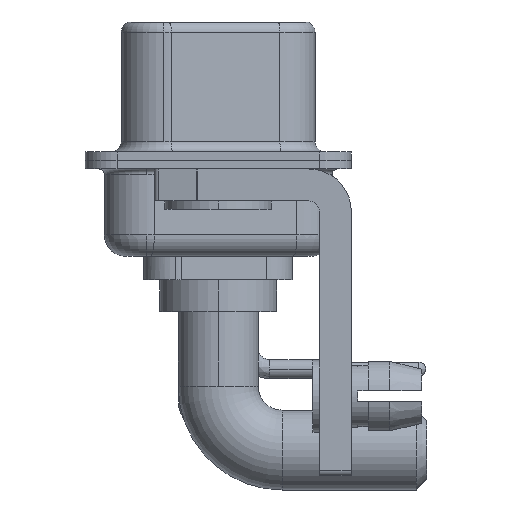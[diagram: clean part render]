
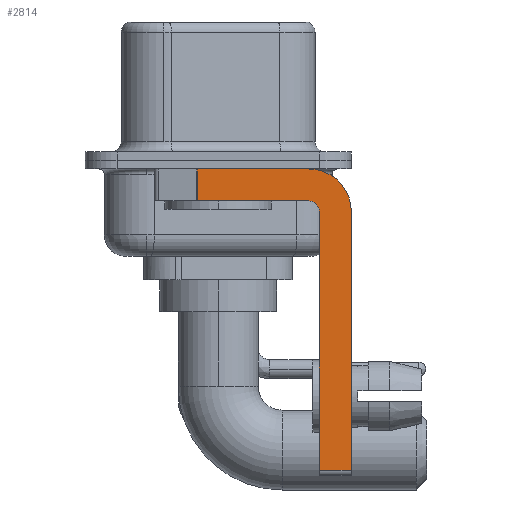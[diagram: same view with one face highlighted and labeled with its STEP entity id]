
A CAD part, left-side view. The second image highlights one B-rep face of the part: STEP entity #2814.
In plain terms, the highlighted planar face has unit normal (-1, 0, 0).
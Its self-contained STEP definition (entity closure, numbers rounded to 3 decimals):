
#138 = CARTESIAN_POINT ( 'NONE',  ( -2.9, -4.25, -1.9 ) ) ;
#366 = VERTEX_POINT ( 'NONE', #13145 ) ;
#1314 = EDGE_CURVE ( 'NONE', #11396, #16834, #12410, .T. ) ;
#1599 = VECTOR ( 'NONE', #16602, 1000. ) ;
#1922 = ORIENTED_EDGE ( 'NONE', *, *, #1314, .F. ) ;
#2042 = DIRECTION ( 'NONE',  ( -1., 0., 0. ) ) ;
#2145 = ORIENTED_EDGE ( 'NONE', *, *, #15794, .T. ) ;
#2553 = DIRECTION ( 'NONE',  ( 0., 0., -1. ) ) ;
#2814 = ADVANCED_FACE ( 'NONE', ( #3043 ), #17117, .F. ) ;
#2923 = CARTESIAN_POINT ( 'NONE',  ( -2.9, -4.75, -2.4 ) ) ;
#3043 = FACE_OUTER_BOUND ( 'NONE', #11314, .T. ) ;
#3869 = DIRECTION ( 'NONE',  ( 0., 0., 1. ) ) ;
#4342 = EDGE_CURVE ( 'NONE', #366, #18215, #15462, .T. ) ;
#4359 = LINE ( 'NONE', #24455, #23652 ) ;
#4376 = ORIENTED_EDGE ( 'NONE', *, *, #16772, .T. ) ;
#4397 = CARTESIAN_POINT ( 'NONE',  ( -2.9, -6.25, -2.4 ) ) ;
#5272 = CARTESIAN_POINT ( 'NONE',  ( -2.9, -4.25, -2.4 ) ) ;
#6816 = CIRCLE ( 'NONE', #10605, 0.5 ) ;
#7728 = EDGE_CURVE ( 'NONE', #23266, #24314, #14425, .T. ) ;
#7977 = DIRECTION ( 'NONE',  ( 0., 0., -1. ) ) ;
#9319 = VECTOR ( 'NONE', #7977, 1000. ) ;
#9496 = VECTOR ( 'NONE', #2553, 1000. ) ;
#9555 = CARTESIAN_POINT ( 'NONE',  ( -2.9, 0.978, -1.9 ) ) ;
#9765 = CARTESIAN_POINT ( 'NONE',  ( -2.9, -6.25, -14.55 ) ) ;
#10085 = DIRECTION ( 'NONE',  ( 0., 0., 1. ) ) ;
#10206 = ORIENTED_EDGE ( 'NONE', *, *, #22269, .F. ) ;
#10605 = AXIS2_PLACEMENT_3D ( 'NONE', #22157, #2042, #10085 ) ;
#11314 = EDGE_LOOP ( 'NONE', ( #15581, #4376, #1922, #10206, #14686, #2145, #24865, #20052 ) ) ;
#11396 = VERTEX_POINT ( 'NONE', #138 ) ;
#11513 = CARTESIAN_POINT ( 'NONE',  ( -2.9, -4.75, -14.8 ) ) ;
#11521 = CARTESIAN_POINT ( 'NONE',  ( -2.9, 0.978, -1.9 ) ) ;
#11612 = DIRECTION ( 'NONE',  ( 1., 0., 0. ) ) ;
#11923 = CARTESIAN_POINT ( 'NONE',  ( -2.9, -4.25, -14.55 ) ) ;
#12410 = LINE ( 'NONE', #14649, #1599 ) ;
#13058 = DIRECTION ( 'NONE',  ( 0., 0., -1. ) ) ;
#13145 = CARTESIAN_POINT ( 'NONE',  ( -2.9, -4.75, -14.55 ) ) ;
#13555 = AXIS2_PLACEMENT_3D ( 'NONE', #15718, #21760, #23703 ) ;
#14024 = LINE ( 'NONE', #9555, #9319 ) ;
#14383 = CARTESIAN_POINT ( 'NONE',  ( -2.9, -6.25, -2.4 ) ) ;
#14425 = LINE ( 'NONE', #4397, #9496 ) ;
#14466 = VECTOR ( 'NONE', #3869, 1000. ) ;
#14649 = CARTESIAN_POINT ( 'NONE',  ( -2.9, -4.25, -1.9 ) ) ;
#14686 = ORIENTED_EDGE ( 'NONE', *, *, #4342, .F. ) ;
#15462 = LINE ( 'NONE', #11513, #14466 ) ;
#15581 = ORIENTED_EDGE ( 'NONE', *, *, #18548, .F. ) ;
#15718 = CARTESIAN_POINT ( 'NONE',  ( -2.9, -4.25, -2.4 ) ) ;
#15794 = EDGE_CURVE ( 'NONE', #366, #24314, #17681, .T. ) ;
#16602 = DIRECTION ( 'NONE',  ( 0., 1., 0. ) ) ;
#16772 = EDGE_CURVE ( 'NONE', #24052, #16834, #14024, .T. ) ;
#16834 = VERTEX_POINT ( 'NONE', #11521 ) ;
#17117 = PLANE ( 'NONE',  #19473 ) ;
#17681 = LINE ( 'NONE', #11923, #19765 ) ;
#17827 = DIRECTION ( 'NONE',  ( 0., -1., 0. ) ) ;
#18215 = VERTEX_POINT ( 'NONE', #2923 ) ;
#18546 = CARTESIAN_POINT ( 'NONE',  ( -2.9, -4.25, -0.4 ) ) ;
#18548 = EDGE_CURVE ( 'NONE', #24052, #24475, #4359, .T. ) ;
#18582 = CARTESIAN_POINT ( 'NONE',  ( -2.9, 0.978, -0.4 ) ) ;
#19473 = AXIS2_PLACEMENT_3D ( 'NONE', #5272, #11612, #13058 ) ;
#19765 = VECTOR ( 'NONE', #17827, 1000. ) ;
#20052 = ORIENTED_EDGE ( 'NONE', *, *, #20947, .F. ) ;
#20947 = EDGE_CURVE ( 'NONE', #24475, #23266, #24841, .T. ) ;
#21760 = DIRECTION ( 'NONE',  ( 1., 0., 0. ) ) ;
#22157 = CARTESIAN_POINT ( 'NONE',  ( -2.9, -4.25, -2.4 ) ) ;
#22269 = EDGE_CURVE ( 'NONE', #18215, #11396, #6816, .T. ) ;
#22510 = DIRECTION ( 'NONE',  ( 0., -1., 0. ) ) ;
#23266 = VERTEX_POINT ( 'NONE', #14383 ) ;
#23652 = VECTOR ( 'NONE', #22510, 1000. ) ;
#23703 = DIRECTION ( 'NONE',  ( 0., 0., -1. ) ) ;
#24052 = VERTEX_POINT ( 'NONE', #18582 ) ;
#24314 = VERTEX_POINT ( 'NONE', #9765 ) ;
#24455 = CARTESIAN_POINT ( 'NONE',  ( -2.9, 3., -0.4 ) ) ;
#24475 = VERTEX_POINT ( 'NONE', #18546 ) ;
#24841 = CIRCLE ( 'NONE', #13555, 2. ) ;
#24865 = ORIENTED_EDGE ( 'NONE', *, *, #7728, .F. ) ;
